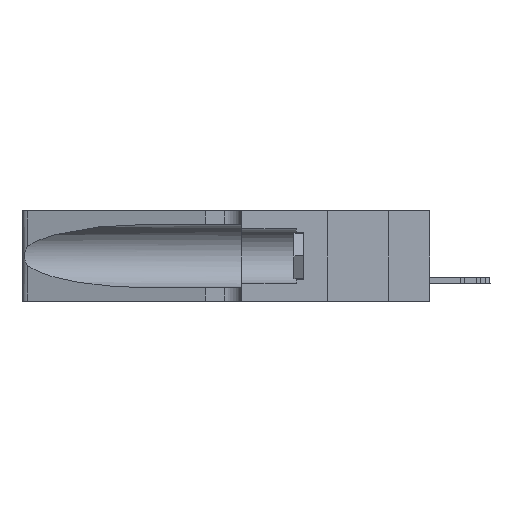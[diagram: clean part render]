
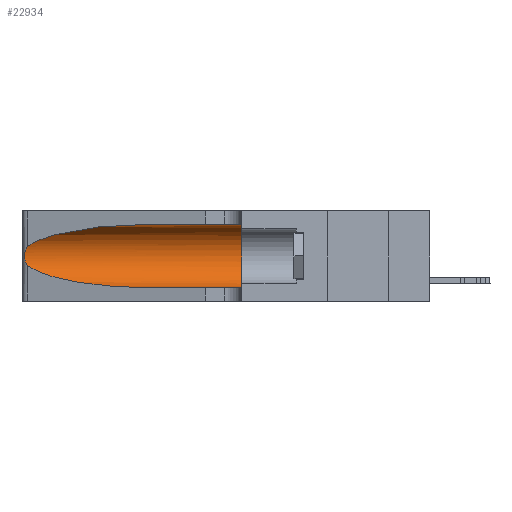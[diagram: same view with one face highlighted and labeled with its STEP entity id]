
A CAD part, left-side view. The second image highlights one B-rep face of the part: STEP entity #22934.
In plain terms, the highlighted cylindrical face has radius 3.308 mm (diameter 6.617 mm), a partial arc.
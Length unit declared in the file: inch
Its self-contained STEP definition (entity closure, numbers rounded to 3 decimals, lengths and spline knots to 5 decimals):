
#1700 = CARTESIAN_POINT ( 'NONE',  ( 0.1305, 0.72297, 0.31525 ) ) ;
#2511 = CARTESIAN_POINT ( 'NONE',  ( 0.25487, 1.22718, 0.22369 ) ) ;
#2886 = CARTESIAN_POINT ( 'NONE',  ( 0.1305, 1.61858, 0.05475 ) ) ;
#2991 = EDGE_CURVE ( 'NONE', #10299, #13897, #5509, .T. ) ;
#3747 = ORIENTED_EDGE ( 'NONE', *, *, #40866, .T. ) ;
#4573 = DIRECTION ( 'NONE',  ( 0., 0., -1. ) ) ;
#5509 = B_SPLINE_CURVE_WITH_KNOTS ( 'NONE', 3,
 ( #2511, #25028, #13762, #29031, #40250, #36306, #21254, #13930, #47827, #10189, #47321, #6604, #28702, #32364 ),
 .UNSPECIFIED., .F., .F.,
 ( 4, 2, 2, 2, 2, 2, 4 ),
 ( 0., 0.00027, 0.00053, 0.00107, 0.0016, 0.00187, 0.00214 ),
 .UNSPECIFIED. ) ;
#6604 = CARTESIAN_POINT ( 'NONE',  ( 0.25639, 1.23186, 0.15144 ) ) ;
#8802 = CARTESIAN_POINT ( 'NONE',  ( 0.1305, 0.72297, 0.05475 ) ) ;
#8957 = CIRCLE ( 'NONE', #19474, 0.13025 ) ;
#8986 = CARTESIAN_POINT ( 'NONE',  ( 0.25487, 1.22718, 0.14631 ) ) ;
#10189 = CARTESIAN_POINT ( 'NONE',  ( 0.25856, 1.23593, 0.16098 ) ) ;
#10299 = VERTEX_POINT ( 'NONE', #32361 ) ;
#10615 = CARTESIAN_POINT ( 'NONE',  ( 0.1305, 1.61858, 0.31525 ) ) ;
#11176 = DIRECTION ( 'NONE',  ( 0., -1., 0. ) ) ;
#11747 = DIRECTION ( 'NONE',  ( 0., -1., 0. ) ) ;
#12159 = EDGE_CURVE ( 'NONE', #47679, #31752, #28009, .T. ) ;
#13382 = ORIENTED_EDGE ( 'NONE', *, *, #2991, .T. ) ;
#13762 = CARTESIAN_POINT ( 'NONE',  ( 0.25639, 1.23184, 0.21858 ) ) ;
#13864 = VECTOR ( 'NONE', #11176, 39.37008 ) ;
#13897 = VERTEX_POINT ( 'NONE', #18028 ) ;
#13930 = CARTESIAN_POINT ( 'NONE',  ( 0.26075, 1.23896, 0.178 ) ) ;
#14565 = CARTESIAN_POINT ( 'NONE',  ( 0.18966, 0.96281, 0.31525 ) ) ;
#16112 = ORIENTED_EDGE ( 'NONE', *, *, #36549, .F. ) ;
#16626 = VERTEX_POINT ( 'NONE', #8802 ) ;
#17937 = VERTEX_POINT ( 'NONE', #23330 ) ;
#18028 = CARTESIAN_POINT ( 'NONE',  ( 0.25487, 1.22718, 0.14631 ) ) ;
#19474 = AXIS2_PLACEMENT_3D ( 'NONE', #31660, #20382, #35616 ) ;
#19851 = CARTESIAN_POINT ( 'NONE',  ( 0.2373, 1.15595, 0.08982 ) ) ;
#20048 = AXIS2_PLACEMENT_3D ( 'NONE', #23142, #11747, #4573 ) ;
#20155 = FACE_OUTER_BOUND ( 'NONE', #33178, .T. ) ;
#20382 = DIRECTION ( 'NONE',  ( 0., 1., 0. ) ) ;
#21254 = CARTESIAN_POINT ( 'NONE',  ( 0.26075, 1.23896, 0.19203 ) ) ;
#22934 = ADVANCED_FACE ( 'NONE', ( #20155 ), #23688, .F. ) ;
#23142 = CARTESIAN_POINT ( 'NONE',  ( 0.1305, 1.61858, 0.185 ) ) ;
#23330 = CARTESIAN_POINT ( 'NONE',  ( 0.1305, 0.35, 0.05475 ) ) ;
#23688 = CYLINDRICAL_SURFACE ( 'NONE', #20048, 0.13025 ) ;
#24424 = VECTOR ( 'NONE', #44449, 39.37008 ) ;
#25028 = CARTESIAN_POINT ( 'NONE',  ( 0.25555, 1.22994, 0.2215 ) ) ;
#28009 = LINE ( 'NONE', #10615, #24424 ) ;
#28702 = CARTESIAN_POINT ( 'NONE',  ( 0.25555, 1.22993, 0.14849 ) ) ;
#28928 = ORIENTED_EDGE ( 'NONE', *, *, #12159, .F. ) ;
#29031 = CARTESIAN_POINT ( 'NONE',  ( 0.25787, 1.23484, 0.2124 ) ) ;
#29421 = EDGE_CURVE ( 'NONE', #16626, #17937, #33865, .T. ) ;
#30168 =( BOUNDED_CURVE ( )  B_SPLINE_CURVE ( 3, ( #32843, #14565, #40407, #47969 ),
 .UNSPECIFIED., .F., .T. ) 
 B_SPLINE_CURVE_WITH_KNOTS ( ( 4, 4 ),
 ( 1.5708, 2.84003 ),
 .UNSPECIFIED. ) 
 CURVE ( )  GEOMETRIC_REPRESENTATION_ITEM ( )  RATIONAL_B_SPLINE_CURVE ( ( 1., 0.87, 0.87, 1. ) ) 
 REPRESENTATION_ITEM ( '' )  );
#31660 = CARTESIAN_POINT ( 'NONE',  ( 0.1305, 0.35, 0.185 ) ) ;
#31752 = VERTEX_POINT ( 'NONE', #43338 ) ;
#31808 = EDGE_CURVE ( 'NONE', #47679, #10299, #30168, .T. ) ;
#32361 = CARTESIAN_POINT ( 'NONE',  ( 0.25487, 1.22718, 0.22369 ) ) ;
#32364 = CARTESIAN_POINT ( 'NONE',  ( 0.25487, 1.22718, 0.14631 ) ) ;
#32843 = CARTESIAN_POINT ( 'NONE',  ( 0.1305, 0.72297, 0.31525 ) ) ;
#33178 = EDGE_LOOP ( 'NONE', ( #40679, #13382, #3747, #46153, #16112, #28928 ) ) ;
#33865 = LINE ( 'NONE', #2886, #13864 ) ;
#35616 = DIRECTION ( 'NONE',  ( 0., 0., 1. ) ) ;
#36306 = CARTESIAN_POINT ( 'NONE',  ( 0.26018, 1.23835, 0.19895 ) ) ;
#36549 = EDGE_CURVE ( 'NONE', #31752, #17937, #8957, .T. ) ;
#40250 = CARTESIAN_POINT ( 'NONE',  ( 0.25854, 1.2359, 0.20912 ) ) ;
#40407 = CARTESIAN_POINT ( 'NONE',  ( 0.2373, 1.15595, 0.28018 ) ) ;
#40679 = ORIENTED_EDGE ( 'NONE', *, *, #31808, .T. ) ;
#40866 = EDGE_CURVE ( 'NONE', #13897, #16626, #43476, .T. ) ;
#43338 = CARTESIAN_POINT ( 'NONE',  ( 0.1305, 0.35, 0.31525 ) ) ;
#43476 =( BOUNDED_CURVE ( )  B_SPLINE_CURVE ( 3, ( #8986, #19851, #46251, #46074 ),
 .UNSPECIFIED., .F., .F. ) 
 B_SPLINE_CURVE_WITH_KNOTS ( ( 4, 4 ),
 ( 3.44316, 4.71239 ),
 .UNSPECIFIED. ) 
 CURVE ( )  GEOMETRIC_REPRESENTATION_ITEM ( )  RATIONAL_B_SPLINE_CURVE ( ( 1., 0.87, 0.87, 1. ) ) 
 REPRESENTATION_ITEM ( '' )  );
#44449 = DIRECTION ( 'NONE',  ( 0., -1., 0. ) ) ;
#46074 = CARTESIAN_POINT ( 'NONE',  ( 0.1305, 0.72297, 0.05475 ) ) ;
#46153 = ORIENTED_EDGE ( 'NONE', *, *, #29421, .T. ) ;
#46251 = CARTESIAN_POINT ( 'NONE',  ( 0.18966, 0.96281, 0.05475 ) ) ;
#47321 = CARTESIAN_POINT ( 'NONE',  ( 0.25789, 1.23486, 0.15765 ) ) ;
#47679 = VERTEX_POINT ( 'NONE', #1700 ) ;
#47827 = CARTESIAN_POINT ( 'NONE',  ( 0.26017, 1.23833, 0.17102 ) ) ;
#47969 = CARTESIAN_POINT ( 'NONE',  ( 0.25487, 1.22718, 0.22369 ) ) ;
